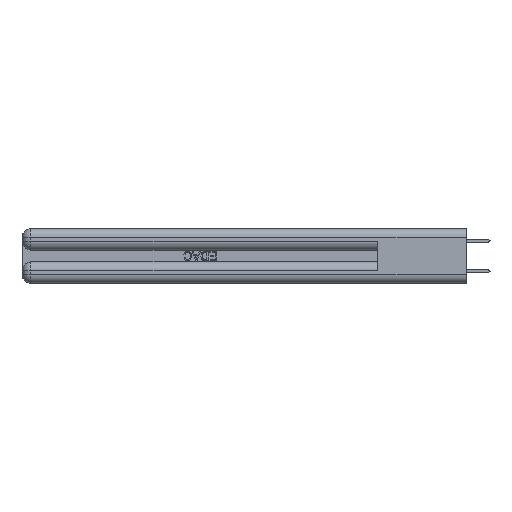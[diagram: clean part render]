
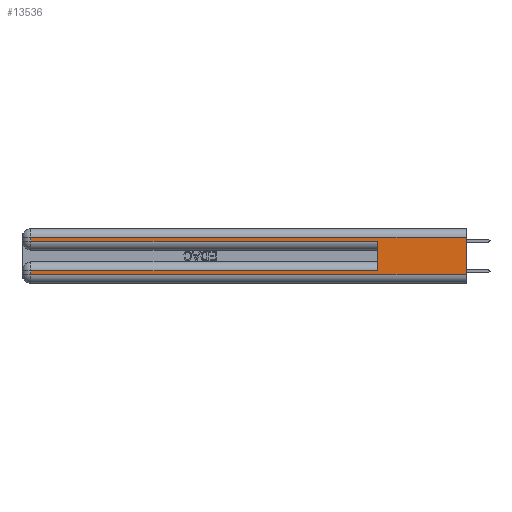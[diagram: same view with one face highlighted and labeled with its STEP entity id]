
A CAD part, left-side view. The second image highlights one B-rep face of the part: STEP entity #13536.
In plain terms, the highlighted planar face has unit normal (-1, 0, 0).
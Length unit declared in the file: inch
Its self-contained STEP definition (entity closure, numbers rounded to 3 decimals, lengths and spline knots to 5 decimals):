
#872 = CARTESIAN_POINT ( 'NONE',  ( 0., 0.6, 0.285 ) ) ;
#1338 = CARTESIAN_POINT ( 'NONE',  ( 0., 2.94, 0.31 ) ) ;
#1479 = EDGE_CURVE ( 'NONE', #6435, #27198, #42262, .T. ) ;
#2327 = CARTESIAN_POINT ( 'NONE',  ( 0., 0., 0.31 ) ) ;
#5230 = LINE ( 'NONE', #27499, #24266 ) ;
#5258 = CARTESIAN_POINT ( 'NONE',  ( 0., 2.94, 0.37 ) ) ;
#5451 = DIRECTION ( 'NONE',  ( 0., 1., 0. ) ) ;
#6023 = EDGE_CURVE ( 'NONE', #24555, #23378, #9133, .T. ) ;
#6435 = VERTEX_POINT ( 'NONE', #1338 ) ;
#6541 = LINE ( 'NONE', #24591, #16672 ) ;
#6682 = CARTESIAN_POINT ( 'NONE',  ( 0., 0.6, 0.085 ) ) ;
#7024 = AXIS2_PLACEMENT_3D ( 'NONE', #20408, #47039, #24254 ) ;
#7332 = ORIENTED_EDGE ( 'NONE', *, *, #33643, .T. ) ;
#8480 = DIRECTION ( 'NONE',  ( 0., 1., 0. ) ) ;
#8706 = EDGE_CURVE ( 'NONE', #29553, #10777, #16478, .T. ) ;
#9072 = DIRECTION ( 'NONE',  ( 0., 0., -1. ) ) ;
#9133 = LINE ( 'NONE', #47972, #44868 ) ;
#10777 = VERTEX_POINT ( 'NONE', #872 ) ;
#12596 = VECTOR ( 'NONE', #9072, 39.37008 ) ;
#12809 = PLANE ( 'NONE',  #7024 ) ;
#13536 = ADVANCED_FACE ( 'NONE', ( #48206 ), #12809, .F. ) ;
#13605 = EDGE_CURVE ( 'NONE', #29553, #48069, #6541, .T. ) ;
#13804 = LINE ( 'NONE', #5258, #12596 ) ;
#14122 = CARTESIAN_POINT ( 'NONE',  ( 0., 0., 0.06 ) ) ;
#14274 = LINE ( 'NONE', #30654, #43386 ) ;
#16471 = VERTEX_POINT ( 'NONE', #44247 ) ;
#16478 = LINE ( 'NONE', #45159, #35527 ) ;
#16672 = VECTOR ( 'NONE', #5451, 39.37008 ) ;
#17144 = CARTESIAN_POINT ( 'NONE',  ( 0., 2.94, 0.285 ) ) ;
#18673 = VECTOR ( 'NONE', #33684, 39.37008 ) ;
#20408 = CARTESIAN_POINT ( 'NONE',  ( 0., 0., 0.37 ) ) ;
#22167 = ORIENTED_EDGE ( 'NONE', *, *, #43047, .T. ) ;
#22962 = ORIENTED_EDGE ( 'NONE', *, *, #27792, .T. ) ;
#23378 = VERTEX_POINT ( 'NONE', #14122 ) ;
#24254 = DIRECTION ( 'NONE',  ( 0., 0., -1. ) ) ;
#24266 = VECTOR ( 'NONE', #8480, 39.37008 ) ;
#24555 = VERTEX_POINT ( 'NONE', #2327 ) ;
#24591 = CARTESIAN_POINT ( 'NONE',  ( 0., 0., 0.085 ) ) ;
#25136 = CARTESIAN_POINT ( 'NONE',  ( 0., 2.94, 0.37 ) ) ;
#25835 = ORIENTED_EDGE ( 'NONE', *, *, #8706, .F. ) ;
#27198 = VERTEX_POINT ( 'NONE', #17144 ) ;
#27499 = CARTESIAN_POINT ( 'NONE',  ( 0., 0., 0.31 ) ) ;
#27792 = EDGE_CURVE ( 'NONE', #48069, #16471, #13804, .T. ) ;
#28847 = LINE ( 'NONE', #37310, #18673 ) ;
#29553 = VERTEX_POINT ( 'NONE', #6682 ) ;
#29865 = EDGE_CURVE ( 'NONE', #24555, #6435, #5230, .T. ) ;
#30099 = DIRECTION ( 'NONE',  ( 0., 0., 1. ) ) ;
#30654 = CARTESIAN_POINT ( 'NONE',  ( 0., 0., 0.06 ) ) ;
#33643 = EDGE_CURVE ( 'NONE', #16471, #23378, #14274, .T. ) ;
#33684 = DIRECTION ( 'NONE',  ( 0., -1., 0. ) ) ;
#34479 = DIRECTION ( 'NONE',  ( 0., -1., 0. ) ) ;
#35516 = ORIENTED_EDGE ( 'NONE', *, *, #29865, .T. ) ;
#35527 = VECTOR ( 'NONE', #30099, 39.37008 ) ;
#35978 = CARTESIAN_POINT ( 'NONE',  ( 0., 2.94, 0.085 ) ) ;
#37310 = CARTESIAN_POINT ( 'NONE',  ( 0., 0., 0.285 ) ) ;
#42262 = LINE ( 'NONE', #25136, #43452 ) ;
#43047 = EDGE_CURVE ( 'NONE', #27198, #10777, #28847, .T. ) ;
#43386 = VECTOR ( 'NONE', #34479, 39.37008 ) ;
#43452 = VECTOR ( 'NONE', #47877, 39.37008 ) ;
#43714 = ORIENTED_EDGE ( 'NONE', *, *, #6023, .F. ) ;
#44247 = CARTESIAN_POINT ( 'NONE',  ( 0., 2.94, 0.06 ) ) ;
#44331 = DIRECTION ( 'NONE',  ( 0., 0., -1. ) ) ;
#44359 = ORIENTED_EDGE ( 'NONE', *, *, #13605, .T. ) ;
#44868 = VECTOR ( 'NONE', #44331, 39.37008 ) ;
#45159 = CARTESIAN_POINT ( 'NONE',  ( 0., 0.6, 0.145 ) ) ;
#47039 = DIRECTION ( 'NONE',  ( 1., 0., 0. ) ) ;
#47399 = ORIENTED_EDGE ( 'NONE', *, *, #1479, .T. ) ;
#47877 = DIRECTION ( 'NONE',  ( 0., 0., -1. ) ) ;
#47972 = CARTESIAN_POINT ( 'NONE',  ( 0., 0., 0.37 ) ) ;
#48069 = VERTEX_POINT ( 'NONE', #35978 ) ;
#48206 = FACE_OUTER_BOUND ( 'NONE', #48336, .T. ) ;
#48336 = EDGE_LOOP ( 'NONE', ( #43714, #35516, #47399, #22167, #25835, #44359, #22962, #7332 ) ) ;
